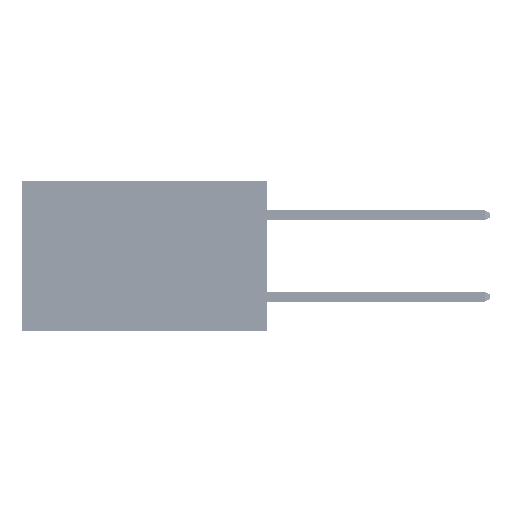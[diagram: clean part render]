
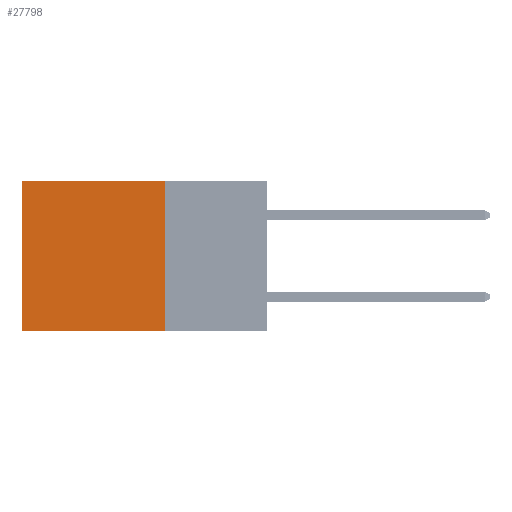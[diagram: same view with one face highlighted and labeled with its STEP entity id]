
A CAD part, left-side view. The second image highlights one B-rep face of the part: STEP entity #27798.
In plain terms, the highlighted planar face has unit normal (-1, 0, 0).
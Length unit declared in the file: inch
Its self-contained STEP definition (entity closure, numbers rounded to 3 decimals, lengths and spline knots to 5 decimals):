
#646 = DIRECTION ( 'NONE',  ( 0., 1., 0. ) ) ;
#1045 = LINE ( 'NONE', #37175, #10418 ) ;
#2884 = VECTOR ( 'NONE', #646, 39.37008 ) ;
#3964 = LINE ( 'NONE', #34725, #24074 ) ;
#5380 = LINE ( 'NONE', #36725, #2884 ) ;
#6289 = CARTESIAN_POINT ( 'NONE',  ( 0.2875, 0.6, 0. ) ) ;
#7530 = CARTESIAN_POINT ( 'NONE',  ( 0.2875, 0.25, 0. ) ) ;
#10418 = VECTOR ( 'NONE', #21276, 39.37008 ) ;
#13573 = EDGE_LOOP ( 'NONE', ( #41213, #26158, #45830, #36342 ) ) ;
#15638 = PLANE ( 'NONE',  #48467 ) ;
#17662 = EDGE_CURVE ( 'NONE', #50917, #51223, #5380, .T. ) ;
#18168 = CARTESIAN_POINT ( 'NONE',  ( 0.2875, 0.6, -0.37 ) ) ;
#19675 = DIRECTION ( 'NONE',  ( 1., 0., 0. ) ) ;
#20040 = CARTESIAN_POINT ( 'NONE',  ( 0.2875, 0.25, -0.37 ) ) ;
#21276 = DIRECTION ( 'NONE',  ( 0., 0., -1. ) ) ;
#24074 = VECTOR ( 'NONE', #42395, 39.37008 ) ;
#24309 = VERTEX_POINT ( 'NONE', #20040 ) ;
#24391 = CARTESIAN_POINT ( 'NONE',  ( 0.2875, 0.25, 0. ) ) ;
#26158 = ORIENTED_EDGE ( 'NONE', *, *, #29639, .F. ) ;
#27798 = ADVANCED_FACE ( 'NONE', ( #42865 ), #15638, .F. ) ;
#29370 = DIRECTION ( 'NONE',  ( 0., 0., -1. ) ) ;
#29639 = EDGE_CURVE ( 'NONE', #24309, #32468, #3964, .T. ) ;
#32335 = EDGE_CURVE ( 'NONE', #50917, #24309, #33869, .T. ) ;
#32468 = VERTEX_POINT ( 'NONE', #18168 ) ;
#33869 = LINE ( 'NONE', #49196, #43225 ) ;
#34415 = EDGE_CURVE ( 'NONE', #51223, #32468, #1045, .T. ) ;
#34725 = CARTESIAN_POINT ( 'NONE',  ( 0.2875, 0.25, -0.37 ) ) ;
#36342 = ORIENTED_EDGE ( 'NONE', *, *, #17662, .T. ) ;
#36725 = CARTESIAN_POINT ( 'NONE',  ( 0.2875, 0.25, 0. ) ) ;
#37175 = CARTESIAN_POINT ( 'NONE',  ( 0.2875, 0.6, 0. ) ) ;
#41213 = ORIENTED_EDGE ( 'NONE', *, *, #34415, .T. ) ;
#42395 = DIRECTION ( 'NONE',  ( 0., 1., 0. ) ) ;
#42865 = FACE_OUTER_BOUND ( 'NONE', #13573, .T. ) ;
#43225 = VECTOR ( 'NONE', #29370, 39.37008 ) ;
#45830 = ORIENTED_EDGE ( 'NONE', *, *, #32335, .F. ) ;
#47583 = DIRECTION ( 'NONE',  ( 0., 0., -1. ) ) ;
#48467 = AXIS2_PLACEMENT_3D ( 'NONE', #7530, #19675, #47583 ) ;
#49196 = CARTESIAN_POINT ( 'NONE',  ( 0.2875, 0.25, 0. ) ) ;
#50917 = VERTEX_POINT ( 'NONE', #24391 ) ;
#51223 = VERTEX_POINT ( 'NONE', #6289 ) ;
